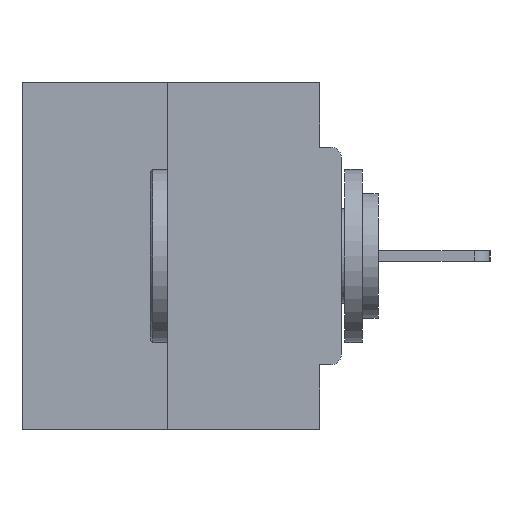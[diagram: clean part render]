
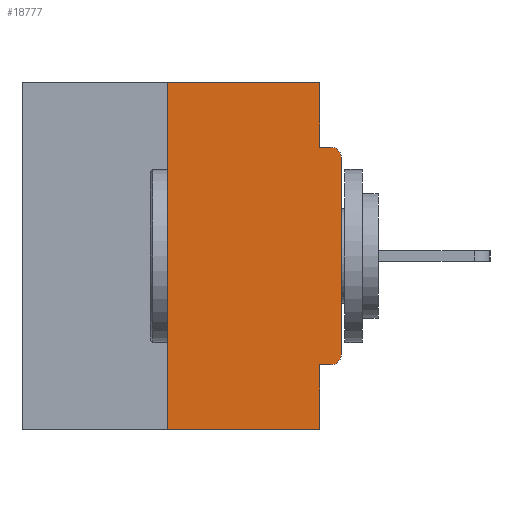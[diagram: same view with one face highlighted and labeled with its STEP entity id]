
A CAD part, left-side view. The second image highlights one B-rep face of the part: STEP entity #18777.
In plain terms, the highlighted planar face has unit normal (-1, 0, 0).
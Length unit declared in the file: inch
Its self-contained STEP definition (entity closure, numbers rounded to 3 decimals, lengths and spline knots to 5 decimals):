
#217 = VECTOR ( 'NONE', #2041, 39.37008 ) ;
#393 = VECTOR ( 'NONE', #21081, 39.37008 ) ;
#443 = LINE ( 'NONE', #27397, #21847 ) ;
#1513 = CARTESIAN_POINT ( 'NONE',  ( 0., 0.25, -0.5 ) ) ;
#1651 = EDGE_CURVE ( 'NONE', #9032, #22869, #4864, .T. ) ;
#1964 = CARTESIAN_POINT ( 'NONE',  ( 0., 0.031, -0.0935 ) ) ;
#2041 = DIRECTION ( 'NONE',  ( 0., 0., -1. ) ) ;
#2077 = VERTEX_POINT ( 'NONE', #31192 ) ;
#2447 = VERTEX_POINT ( 'NONE', #1964 ) ;
#3933 = VECTOR ( 'NONE', #18767, 39.37008 ) ;
#4583 = ORIENTED_EDGE ( 'NONE', *, *, #17264, .F. ) ;
#4726 = CARTESIAN_POINT ( 'NONE',  ( 0., 0.031, -0.4065 ) ) ;
#4864 = LINE ( 'NONE', #6934, #217 ) ;
#5085 = DIRECTION ( 'NONE',  ( 0., 0., -1. ) ) ;
#6006 = CARTESIAN_POINT ( 'NONE',  ( 0., 0.015, -0.4065 ) ) ;
#6356 = DIRECTION ( 'NONE',  ( 0., 0., 1. ) ) ;
#6450 = EDGE_CURVE ( 'NONE', #15575, #22869, #18717, .T. ) ;
#6630 = DIRECTION ( 'NONE',  ( 0., -1., 0. ) ) ;
#6915 = VECTOR ( 'NONE', #27530, 39.37008 ) ;
#6934 = CARTESIAN_POINT ( 'NONE',  ( 0., 0.031, -0.5 ) ) ;
#7258 = PLANE ( 'NONE',  #7528 ) ;
#7528 = AXIS2_PLACEMENT_3D ( 'NONE', #21884, #14690, #12172 ) ;
#8177 = CARTESIAN_POINT ( 'NONE',  ( 0., 0.25, 0. ) ) ;
#8629 = DIRECTION ( 'NONE',  ( 0., 0., -1. ) ) ;
#9032 = VERTEX_POINT ( 'NONE', #4726 ) ;
#9132 = VERTEX_POINT ( 'NONE', #9814 ) ;
#9507 = ORIENTED_EDGE ( 'NONE', *, *, #29805, .F. ) ;
#9814 = CARTESIAN_POINT ( 'NONE',  ( 0., 0., -0.1085 ) ) ;
#10094 = CARTESIAN_POINT ( 'NONE',  ( 0., 0.031, 0. ) ) ;
#10312 = EDGE_CURVE ( 'NONE', #20214, #9032, #20847, .T. ) ;
#10407 = LINE ( 'NONE', #29768, #18566 ) ;
#10670 = LINE ( 'NONE', #25270, #12016 ) ;
#10862 = DIRECTION ( 'NONE',  ( -1., 0., 0. ) ) ;
#11687 = CARTESIAN_POINT ( 'NONE',  ( 0., 0.031, 0. ) ) ;
#12016 = VECTOR ( 'NONE', #6356, 39.37008 ) ;
#12172 = DIRECTION ( 'NONE',  ( 0., 0., -1. ) ) ;
#12319 = DIRECTION ( 'NONE',  ( 0., 0., 1. ) ) ;
#12440 = CARTESIAN_POINT ( 'NONE',  ( 0., 0., -0.0935 ) ) ;
#13927 = CARTESIAN_POINT ( 'NONE',  ( 0., 0.46, -0.5 ) ) ;
#14690 = DIRECTION ( 'NONE',  ( 1., 0., 0. ) ) ;
#15389 = CARTESIAN_POINT ( 'NONE',  ( 0., 0.031, -0.5 ) ) ;
#15575 = VERTEX_POINT ( 'NONE', #1513 ) ;
#16026 = ORIENTED_EDGE ( 'NONE', *, *, #29406, .T. ) ;
#16457 = LINE ( 'NONE', #11687, #393 ) ;
#16554 = AXIS2_PLACEMENT_3D ( 'NONE', #27675, #10862, #8629 ) ;
#16719 = EDGE_CURVE ( 'NONE', #2447, #26037, #29745, .T. ) ;
#16729 = ORIENTED_EDGE ( 'NONE', *, *, #21994, .T. ) ;
#16869 = EDGE_CURVE ( 'NONE', #9132, #26037, #17082, .T. ) ;
#17082 = CIRCLE ( 'NONE', #16554, 0.015 ) ;
#17264 = EDGE_CURVE ( 'NONE', #15575, #23694, #10670, .T. ) ;
#17352 = ORIENTED_EDGE ( 'NONE', *, *, #16719, .F. ) ;
#18566 = VECTOR ( 'NONE', #25958, 39.37008 ) ;
#18717 = LINE ( 'NONE', #13927, #19899 ) ;
#18767 = DIRECTION ( 'NONE',  ( 0., 1., 0. ) ) ;
#18777 = ADVANCED_FACE ( 'NONE', ( #29316 ), #7258, .F. ) ;
#19647 = VERTEX_POINT ( 'NONE', #10094 ) ;
#19849 = ORIENTED_EDGE ( 'NONE', *, *, #10312, .F. ) ;
#19884 = DIRECTION ( 'NONE',  ( -1., 0., 0. ) ) ;
#19899 = VECTOR ( 'NONE', #6630, 39.37008 ) ;
#20214 = VERTEX_POINT ( 'NONE', #6006 ) ;
#20847 = LINE ( 'NONE', #28280, #3933 ) ;
#21081 = DIRECTION ( 'NONE',  ( 0., 0., -1. ) ) ;
#21847 = VECTOR ( 'NONE', #12319, 39.37008 ) ;
#21884 = CARTESIAN_POINT ( 'NONE',  ( 0., 0.46, 0. ) ) ;
#21994 = EDGE_CURVE ( 'NONE', #2077, #9132, #443, .T. ) ;
#22674 = CIRCLE ( 'NONE', #24685, 0.015 ) ;
#22869 = VERTEX_POINT ( 'NONE', #15389 ) ;
#23694 = VERTEX_POINT ( 'NONE', #8177 ) ;
#24685 = AXIS2_PLACEMENT_3D ( 'NONE', #27165, #19884, #5085 ) ;
#25270 = CARTESIAN_POINT ( 'NONE',  ( 0., 0.25, 0. ) ) ;
#25958 = DIRECTION ( 'NONE',  ( 0., -1., 0. ) ) ;
#26037 = VERTEX_POINT ( 'NONE', #29154 ) ;
#26552 = ORIENTED_EDGE ( 'NONE', *, *, #6450, .T. ) ;
#27165 = CARTESIAN_POINT ( 'NONE',  ( 0., 0.015, -0.3915 ) ) ;
#27397 = CARTESIAN_POINT ( 'NONE',  ( 0., 0., 0. ) ) ;
#27530 = DIRECTION ( 'NONE',  ( 0., -1., 0. ) ) ;
#27675 = CARTESIAN_POINT ( 'NONE',  ( 0., 0.015, -0.1085 ) ) ;
#27703 = ORIENTED_EDGE ( 'NONE', *, *, #16869, .T. ) ;
#28280 = CARTESIAN_POINT ( 'NONE',  ( 0., 0., -0.4065 ) ) ;
#29154 = CARTESIAN_POINT ( 'NONE',  ( 0., 0.015, -0.0935 ) ) ;
#29273 = ORIENTED_EDGE ( 'NONE', *, *, #29576, .F. ) ;
#29316 = FACE_OUTER_BOUND ( 'NONE', #29610, .T. ) ;
#29406 = EDGE_CURVE ( 'NONE', #20214, #2077, #22674, .T. ) ;
#29576 = EDGE_CURVE ( 'NONE', #19647, #2447, #16457, .T. ) ;
#29605 = ORIENTED_EDGE ( 'NONE', *, *, #1651, .F. ) ;
#29610 = EDGE_LOOP ( 'NONE', ( #9507, #4583, #26552, #29605, #19849, #16026, #16729, #27703, #17352, #29273 ) ) ;
#29745 = LINE ( 'NONE', #12440, #6915 ) ;
#29768 = CARTESIAN_POINT ( 'NONE',  ( 0., 0.46, 0. ) ) ;
#29805 = EDGE_CURVE ( 'NONE', #23694, #19647, #10407, .T. ) ;
#31192 = CARTESIAN_POINT ( 'NONE',  ( 0., 0., -0.3915 ) ) ;
